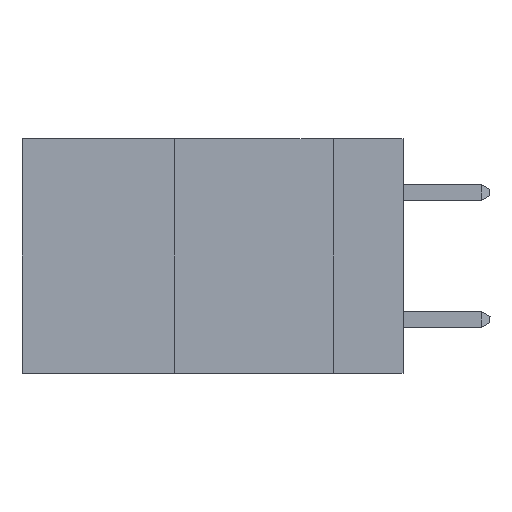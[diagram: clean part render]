
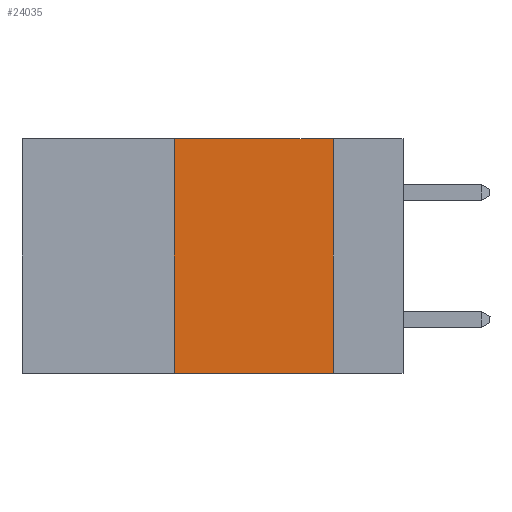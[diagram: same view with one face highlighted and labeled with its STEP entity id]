
A CAD part, left-side view. The second image highlights one B-rep face of the part: STEP entity #24035.
In plain terms, the highlighted planar face has unit normal (-1, 0, 0).
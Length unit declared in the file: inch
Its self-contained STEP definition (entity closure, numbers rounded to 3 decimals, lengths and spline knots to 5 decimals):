
#473 = FACE_OUTER_BOUND ( 'NONE', #8777, .T. ) ;
#2126 = AXIS2_PLACEMENT_3D ( 'NONE', #7288, #24296, #24204 ) ;
#4505 = CARTESIAN_POINT ( 'NONE',  ( 0., 0.36, 0. ) ) ;
#4536 = VECTOR ( 'NONE', #8444, 39.37008 ) ;
#4836 = CARTESIAN_POINT ( 'NONE',  ( 0., 0.6, 0. ) ) ;
#5772 = DIRECTION ( 'NONE',  ( 0., 0., -1. ) ) ;
#6113 = EDGE_CURVE ( 'NONE', #17020, #14402, #13348, .T. ) ;
#6419 = CARTESIAN_POINT ( 'NONE',  ( 0., 0.11, 0. ) ) ;
#7113 = CARTESIAN_POINT ( 'NONE',  ( 0., 0.36, -0.37 ) ) ;
#7212 = PLANE ( 'NONE',  #2126 ) ;
#7288 = CARTESIAN_POINT ( 'NONE',  ( 0., 0.6, 0. ) ) ;
#7335 = ORIENTED_EDGE ( 'NONE', *, *, #8097, .T. ) ;
#7690 = LINE ( 'NONE', #4836, #13861 ) ;
#7772 = LINE ( 'NONE', #21722, #4536 ) ;
#8061 = VECTOR ( 'NONE', #5772, 39.37008 ) ;
#8097 = EDGE_CURVE ( 'NONE', #23170, #14402, #10643, .T. ) ;
#8444 = DIRECTION ( 'NONE',  ( 0., 0., 1. ) ) ;
#8777 = EDGE_LOOP ( 'NONE', ( #24404, #23482, #19433, #7335 ) ) ;
#9611 = CARTESIAN_POINT ( 'NONE',  ( 0., 0.6, -0.37 ) ) ;
#10643 = LINE ( 'NONE', #9611, #23396 ) ;
#11083 = CARTESIAN_POINT ( 'NONE',  ( 0., 0.11, 0. ) ) ;
#12388 = DIRECTION ( 'NONE',  ( 0., -1., 0. ) ) ;
#13348 = LINE ( 'NONE', #11083, #8061 ) ;
#13565 = DIRECTION ( 'NONE',  ( 0., -1., 0. ) ) ;
#13861 = VECTOR ( 'NONE', #12388, 39.37008 ) ;
#14402 = VERTEX_POINT ( 'NONE', #21996 ) ;
#17020 = VERTEX_POINT ( 'NONE', #6419 ) ;
#18795 = VERTEX_POINT ( 'NONE', #4505 ) ;
#18812 = EDGE_CURVE ( 'NONE', #18795, #17020, #7690, .T. ) ;
#19433 = ORIENTED_EDGE ( 'NONE', *, *, #23634, .F. ) ;
#21722 = CARTESIAN_POINT ( 'NONE',  ( 0., 0.36, 0. ) ) ;
#21996 = CARTESIAN_POINT ( 'NONE',  ( 0., 0.11, -0.37 ) ) ;
#23170 = VERTEX_POINT ( 'NONE', #7113 ) ;
#23396 = VECTOR ( 'NONE', #13565, 39.37008 ) ;
#23482 = ORIENTED_EDGE ( 'NONE', *, *, #18812, .F. ) ;
#23634 = EDGE_CURVE ( 'NONE', #23170, #18795, #7772, .T. ) ;
#24035 = ADVANCED_FACE ( 'NONE', ( #473 ), #7212, .F. ) ;
#24204 = DIRECTION ( 'NONE',  ( 0., 0., -1. ) ) ;
#24296 = DIRECTION ( 'NONE',  ( 1., 0., 0. ) ) ;
#24404 = ORIENTED_EDGE ( 'NONE', *, *, #6113, .F. ) ;
